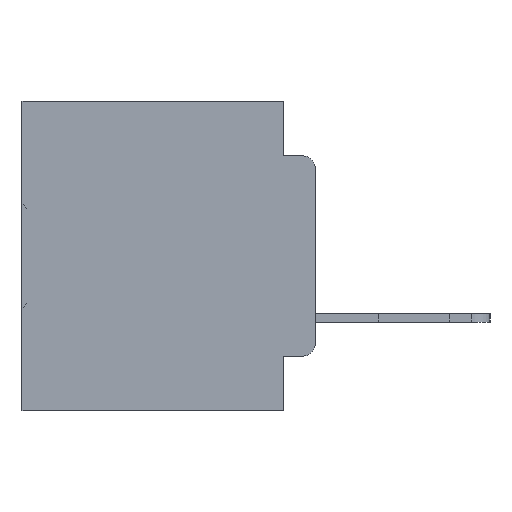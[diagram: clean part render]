
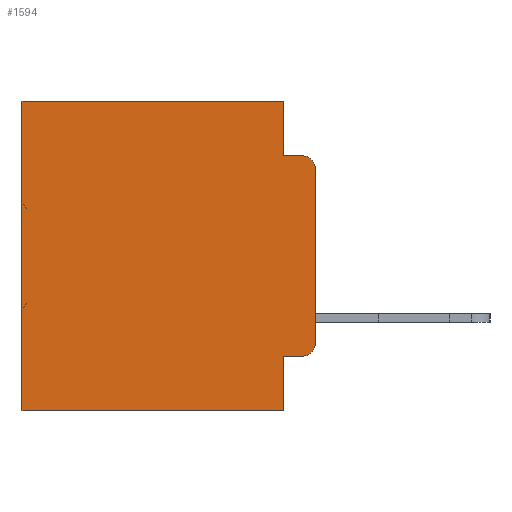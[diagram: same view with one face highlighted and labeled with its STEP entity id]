
A CAD part, left-side view. The second image highlights one B-rep face of the part: STEP entity #1594.
In plain terms, the highlighted planar face has unit normal (-1, 0, 0).
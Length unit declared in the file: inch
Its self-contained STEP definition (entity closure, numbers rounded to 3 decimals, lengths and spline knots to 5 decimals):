
#5 = EDGE_LOOP ( 'NONE', ( #31147, #1156, #19009, #18181, #31382, #17334, #9289, #29756, #8436, #21544 ) ) ;
#561 = EDGE_CURVE ( 'NONE', #27842, #24275, #6995, .T. ) ;
#874 = DIRECTION ( 'NONE',  ( 0., 1., 0. ) ) ;
#924 = LINE ( 'NONE', #15784, #27854 ) ;
#1156 = ORIENTED_EDGE ( 'NONE', *, *, #12182, .T. ) ;
#1434 = DIRECTION ( 'NONE',  ( 0., 1., 0. ) ) ;
#1594 = ADVANCED_FACE ( 'NONE', ( #17096 ), #31905, .F. ) ;
#1863 = CARTESIAN_POINT ( 'NONE',  ( 0.298, 0.473, 0. ) ) ;
#2154 = EDGE_CURVE ( 'NONE', #24275, #30616, #924, .T. ) ;
#2386 = CIRCLE ( 'NONE', #29732, 0.02 ) ;
#2408 = CARTESIAN_POINT ( 'NONE',  ( 0.298, 0.051, 0. ) ) ;
#2567 = VERTEX_POINT ( 'NONE', #19257 ) ;
#2583 = VECTOR ( 'NONE', #20748, 39.37008 ) ;
#3473 = VECTOR ( 'NONE', #13349, 39.37008 ) ;
#3620 = VERTEX_POINT ( 'NONE', #21579 ) ;
#3746 = VECTOR ( 'NONE', #17980, 39.37008 ) ;
#4243 = VECTOR ( 'NONE', #874, 39.37008 ) ;
#6140 = VECTOR ( 'NONE', #27230, 39.37008 ) ;
#6639 = CARTESIAN_POINT ( 'NONE',  ( 0.298, 0.02, -0.3915 ) ) ;
#6830 = CARTESIAN_POINT ( 'NONE',  ( 0.298, 0., 0. ) ) ;
#6995 = LINE ( 'NONE', #2408, #6140 ) ;
#8436 = ORIENTED_EDGE ( 'NONE', *, *, #9676, .T. ) ;
#8676 = CARTESIAN_POINT ( 'NONE',  ( 0.298, 0.051, 0. ) ) ;
#9072 = CARTESIAN_POINT ( 'NONE',  ( 0.298, 0.02, -0.0885 ) ) ;
#9143 = VERTEX_POINT ( 'NONE', #28877 ) ;
#9210 = DIRECTION ( 'NONE',  ( 1., 0., 0. ) ) ;
#9289 = ORIENTED_EDGE ( 'NONE', *, *, #2154, .F. ) ;
#9381 = DIRECTION ( 'NONE',  ( 0., 0., -1. ) ) ;
#9676 = EDGE_CURVE ( 'NONE', #27842, #3620, #25204, .T. ) ;
#9779 = LINE ( 'NONE', #1863, #2583 ) ;
#10332 = VERTEX_POINT ( 'NONE', #26405 ) ;
#10599 = CARTESIAN_POINT ( 'NONE',  ( 0.298, 0., 0. ) ) ;
#11197 = DIRECTION ( 'NONE',  ( 0., -1., 0. ) ) ;
#11695 = CARTESIAN_POINT ( 'NONE',  ( 0.298, 0.02, -0.1085 ) ) ;
#12182 = EDGE_CURVE ( 'NONE', #10332, #28627, #33157, .T. ) ;
#12516 = AXIS2_PLACEMENT_3D ( 'NONE', #6830, #9210, #25297 ) ;
#13349 = DIRECTION ( 'NONE',  ( 0., 0., -1. ) ) ;
#13544 = LINE ( 'NONE', #8676, #27700 ) ;
#14035 = EDGE_CURVE ( 'NONE', #9143, #28627, #24395, .T. ) ;
#14436 = DIRECTION ( 'NONE',  ( 0., 0., -1. ) ) ;
#15155 = EDGE_CURVE ( 'NONE', #3620, #26654, #2386, .T. ) ;
#15193 = CARTESIAN_POINT ( 'NONE',  ( 0.298, 0.051, -0.4115 ) ) ;
#15784 = CARTESIAN_POINT ( 'NONE',  ( 0.298, 0., -0.5 ) ) ;
#17096 = FACE_OUTER_BOUND ( 'NONE', #5, .T. ) ;
#17126 = CARTESIAN_POINT ( 'NONE',  ( 0.298, 0., 0. ) ) ;
#17316 = VECTOR ( 'NONE', #11197, 39.37008 ) ;
#17334 = ORIENTED_EDGE ( 'NONE', *, *, #31774, .T. ) ;
#17980 = DIRECTION ( 'NONE',  ( 0., -1., 0. ) ) ;
#18181 = ORIENTED_EDGE ( 'NONE', *, *, #19403, .F. ) ;
#19009 = ORIENTED_EDGE ( 'NONE', *, *, #14035, .F. ) ;
#19225 = CARTESIAN_POINT ( 'NONE',  ( 0.298, 0.051, -0.0885 ) ) ;
#19257 = CARTESIAN_POINT ( 'NONE',  ( 0.298, 0.051, 0. ) ) ;
#19403 = EDGE_CURVE ( 'NONE', #2567, #9143, #13544, .T. ) ;
#20748 = DIRECTION ( 'NONE',  ( 0., 0., -1. ) ) ;
#21544 = ORIENTED_EDGE ( 'NONE', *, *, #15155, .T. ) ;
#21579 = CARTESIAN_POINT ( 'NONE',  ( 0.298, 0.02, -0.4115 ) ) ;
#22046 = CARTESIAN_POINT ( 'NONE',  ( 0.298, 0.051, -0.5 ) ) ;
#24099 = LINE ( 'NONE', #10599, #3473 ) ;
#24138 = CARTESIAN_POINT ( 'NONE',  ( 0.298, 0.473, 0. ) ) ;
#24275 = VERTEX_POINT ( 'NONE', #22046 ) ;
#24395 = LINE ( 'NONE', #19225, #17316 ) ;
#25204 = LINE ( 'NONE', #33793, #3746 ) ;
#25297 = DIRECTION ( 'NONE',  ( 0., 0., -1. ) ) ;
#25448 = DIRECTION ( 'NONE',  ( -1., 0., 0. ) ) ;
#26405 = CARTESIAN_POINT ( 'NONE',  ( 0.298, 0., -0.1085 ) ) ;
#26654 = VERTEX_POINT ( 'NONE', #28157 ) ;
#27230 = DIRECTION ( 'NONE',  ( 0., 0., -1. ) ) ;
#27417 = DIRECTION ( 'NONE',  ( 0., 0., -1. ) ) ;
#27700 = VECTOR ( 'NONE', #27417, 39.37008 ) ;
#27842 = VERTEX_POINT ( 'NONE', #15193 ) ;
#27854 = VECTOR ( 'NONE', #1434, 39.37008 ) ;
#28157 = CARTESIAN_POINT ( 'NONE',  ( 0.298, 0., -0.3915 ) ) ;
#28575 = AXIS2_PLACEMENT_3D ( 'NONE', #11695, #30331, #14436 ) ;
#28627 = VERTEX_POINT ( 'NONE', #9072 ) ;
#28877 = CARTESIAN_POINT ( 'NONE',  ( 0.298, 0.051, -0.0885 ) ) ;
#29732 = AXIS2_PLACEMENT_3D ( 'NONE', #6639, #25448, #9381 ) ;
#29756 = ORIENTED_EDGE ( 'NONE', *, *, #561, .F. ) ;
#30331 = DIRECTION ( 'NONE',  ( -1., 0., 0. ) ) ;
#30616 = VERTEX_POINT ( 'NONE', #33973 ) ;
#31147 = ORIENTED_EDGE ( 'NONE', *, *, #32447, .F. ) ;
#31382 = ORIENTED_EDGE ( 'NONE', *, *, #32173, .T. ) ;
#31774 = EDGE_CURVE ( 'NONE', #31972, #30616, #9779, .T. ) ;
#31849 = LINE ( 'NONE', #17126, #4243 ) ;
#31905 = PLANE ( 'NONE',  #12516 ) ;
#31972 = VERTEX_POINT ( 'NONE', #24138 ) ;
#32173 = EDGE_CURVE ( 'NONE', #2567, #31972, #31849, .T. ) ;
#32447 = EDGE_CURVE ( 'NONE', #10332, #26654, #24099, .T. ) ;
#33157 = CIRCLE ( 'NONE', #28575, 0.02 ) ;
#33793 = CARTESIAN_POINT ( 'NONE',  ( 0.298, 0.051, -0.4115 ) ) ;
#33973 = CARTESIAN_POINT ( 'NONE',  ( 0.298, 0.473, -0.5 ) ) ;
